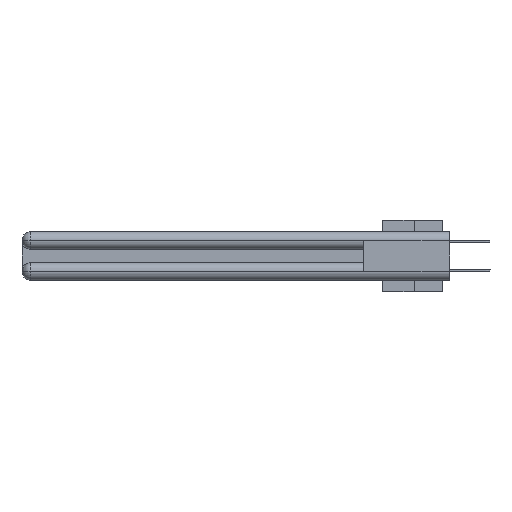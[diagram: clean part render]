
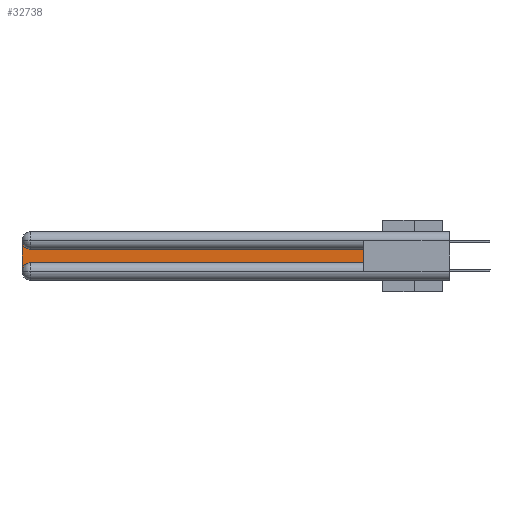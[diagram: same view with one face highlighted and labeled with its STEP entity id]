
A CAD part, left-side view. The second image highlights one B-rep face of the part: STEP entity #32738.
In plain terms, the highlighted planar face has unit normal (-1, 0, 0).
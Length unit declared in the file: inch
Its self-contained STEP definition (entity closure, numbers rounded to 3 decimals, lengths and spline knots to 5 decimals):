
#1893 = CARTESIAN_POINT ( 'NONE',  ( 0.075, 3., -0.0625 ) ) ;
#1922 = ORIENTED_EDGE ( 'NONE', *, *, #27051, .T. ) ;
#4099 = EDGE_CURVE ( 'NONE', #27461, #31899, #21436, .T. ) ;
#4288 = CARTESIAN_POINT ( 'NONE',  ( 0.075, 2.94, -0.2775 ) ) ;
#4411 = VECTOR ( 'NONE', #12544, 39.37008 ) ;
#4890 = CARTESIAN_POINT ( 'NONE',  ( 0.075, 0.6, -0.1225 ) ) ;
#5091 = VERTEX_POINT ( 'NONE', #16861 ) ;
#6222 = CARTESIAN_POINT ( 'NONE',  ( 0.075, 0.6, -0.2175 ) ) ;
#6483 = CARTESIAN_POINT ( 'NONE',  ( 0.075, 0.6, -0.2175 ) ) ;
#8021 = ORIENTED_EDGE ( 'NONE', *, *, #40738, .T. ) ;
#9608 = AXIS2_PLACEMENT_3D ( 'NONE', #21342, #11461, #21755 ) ;
#10886 = PLANE ( 'NONE',  #38296 ) ;
#11461 = DIRECTION ( 'NONE',  ( 1., 0., 0. ) ) ;
#11797 = EDGE_CURVE ( 'NONE', #38234, #27461, #31632, .T. ) ;
#12544 = DIRECTION ( 'NONE',  ( 0., -1., 0. ) ) ;
#12820 = CIRCLE ( 'NONE', #35898, 0.06 ) ;
#13955 = ORIENTED_EDGE ( 'NONE', *, *, #22138, .T. ) ;
#14458 = ORIENTED_EDGE ( 'NONE', *, *, #34848, .T. ) ;
#16173 = LINE ( 'NONE', #6483, #22871 ) ;
#16656 = EDGE_LOOP ( 'NONE', ( #23608, #20378, #8021, #13955, #1922, #14458 ) ) ;
#16861 = CARTESIAN_POINT ( 'NONE',  ( 0.075, 2.94, -0.2175 ) ) ;
#19070 = DIRECTION ( 'NONE',  ( 0., 0., 1. ) ) ;
#20378 = ORIENTED_EDGE ( 'NONE', *, *, #4099, .T. ) ;
#21342 = CARTESIAN_POINT ( 'NONE',  ( 0.075, 2.94, -0.0625 ) ) ;
#21436 = CIRCLE ( 'NONE', #9608, 0.06 ) ;
#21741 = DIRECTION ( 'NONE',  ( 0., 1., 0. ) ) ;
#21755 = DIRECTION ( 'NONE',  ( 0., 0., -1. ) ) ;
#22138 = EDGE_CURVE ( 'NONE', #36996, #5091, #12820, .T. ) ;
#22352 = CARTESIAN_POINT ( 'NONE',  ( 0.075, 0.6, -0.1225 ) ) ;
#22637 = LINE ( 'NONE', #31509, #4411 ) ;
#22871 = VECTOR ( 'NONE', #19070, 39.37008 ) ;
#23468 = DIRECTION ( 'NONE',  ( 1., 0., 0. ) ) ;
#23608 = ORIENTED_EDGE ( 'NONE', *, *, #11797, .T. ) ;
#23669 = CARTESIAN_POINT ( 'NONE',  ( 0.075, 3., -0.1225 ) ) ;
#24880 = CARTESIAN_POINT ( 'NONE',  ( 0.075, 2.94, -0.1225 ) ) ;
#25828 = CARTESIAN_POINT ( 'NONE',  ( 0.075, 3., -0.2175 ) ) ;
#26442 = DIRECTION ( 'NONE',  ( 0., 0., -1. ) ) ;
#27051 = EDGE_CURVE ( 'NONE', #5091, #39211, #22637, .T. ) ;
#27334 = VECTOR ( 'NONE', #21741, 39.37008 ) ;
#27461 = VERTEX_POINT ( 'NONE', #24880 ) ;
#31509 = CARTESIAN_POINT ( 'NONE',  ( 0.075, 0.6, -0.2175 ) ) ;
#31632 = LINE ( 'NONE', #22352, #27334 ) ;
#31899 = VERTEX_POINT ( 'NONE', #1893 ) ;
#32416 = LINE ( 'NONE', #25828, #36304 ) ;
#32738 = ADVANCED_FACE ( 'NONE', ( #39160 ), #10886, .F. ) ;
#33162 = DIRECTION ( 'NONE',  ( 1., 0., 0. ) ) ;
#34848 = EDGE_CURVE ( 'NONE', #39211, #38234, #16173, .T. ) ;
#35898 = AXIS2_PLACEMENT_3D ( 'NONE', #4288, #33162, #39172 ) ;
#36062 = DIRECTION ( 'NONE',  ( 0., 0., -1. ) ) ;
#36304 = VECTOR ( 'NONE', #26442, 39.37008 ) ;
#36996 = VERTEX_POINT ( 'NONE', #40252 ) ;
#38234 = VERTEX_POINT ( 'NONE', #4890 ) ;
#38296 = AXIS2_PLACEMENT_3D ( 'NONE', #23669, #23468, #36062 ) ;
#39160 = FACE_OUTER_BOUND ( 'NONE', #16656, .T. ) ;
#39172 = DIRECTION ( 'NONE',  ( 0., 0., -1. ) ) ;
#39211 = VERTEX_POINT ( 'NONE', #6222 ) ;
#40252 = CARTESIAN_POINT ( 'NONE',  ( 0.075, 3., -0.2775 ) ) ;
#40738 = EDGE_CURVE ( 'NONE', #31899, #36996, #32416, .T. ) ;
